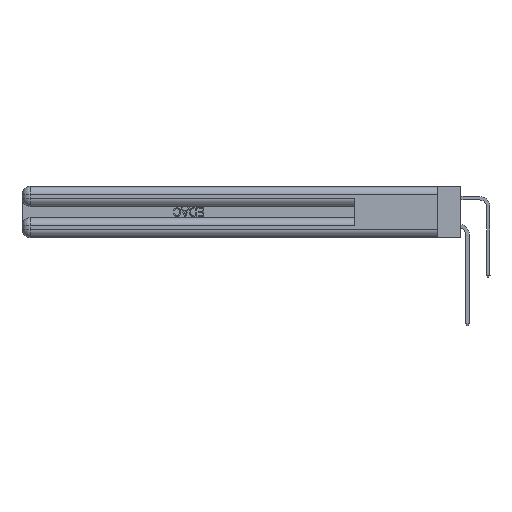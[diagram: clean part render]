
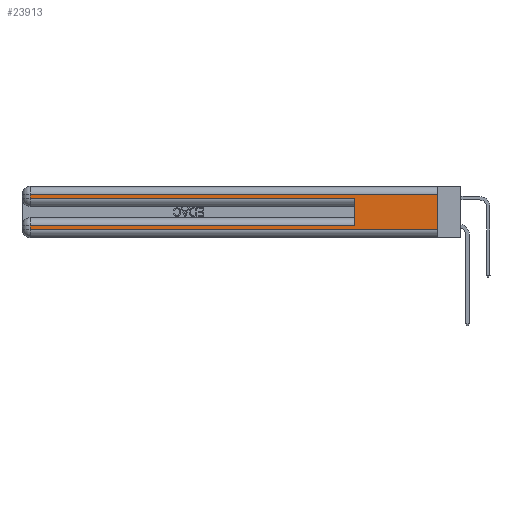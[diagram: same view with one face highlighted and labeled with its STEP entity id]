
A CAD part, left-side view. The second image highlights one B-rep face of the part: STEP entity #23913.
In plain terms, the highlighted planar face has unit normal (-1, 0, 0).
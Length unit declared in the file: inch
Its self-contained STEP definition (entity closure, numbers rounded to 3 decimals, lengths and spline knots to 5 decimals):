
#74 = LINE ( 'NONE', #33646, #19647 ) ;
#191 = CARTESIAN_POINT ( 'NONE',  ( 0., 0.6, 0.145 ) ) ;
#986 = CARTESIAN_POINT ( 'NONE',  ( 0., 2.94, 0.37 ) ) ;
#1189 = VERTEX_POINT ( 'NONE', #39160 ) ;
#1204 = LINE ( 'NONE', #39569, #29414 ) ;
#1362 = VECTOR ( 'NONE', #29673, 39.37008 ) ;
#2371 = CARTESIAN_POINT ( 'NONE',  ( 0., 0., 0.37 ) ) ;
#3102 = DIRECTION ( 'NONE',  ( 0., -1., 0. ) ) ;
#3988 = ORIENTED_EDGE ( 'NONE', *, *, #10481, .T. ) ;
#4118 = CARTESIAN_POINT ( 'NONE',  ( 0., 0., 0.37 ) ) ;
#4418 = ORIENTED_EDGE ( 'NONE', *, *, #36974, .F. ) ;
#5201 = VECTOR ( 'NONE', #18088, 39.37008 ) ;
#7004 = CARTESIAN_POINT ( 'NONE',  ( 0., 0., 0.31 ) ) ;
#8142 = VERTEX_POINT ( 'NONE', #42948 ) ;
#8772 = CARTESIAN_POINT ( 'NONE',  ( 0., 0.6, 0.285 ) ) ;
#9786 = PLANE ( 'NONE',  #21915 ) ;
#10060 = EDGE_CURVE ( 'NONE', #22740, #30011, #74, .T. ) ;
#10203 = VECTOR ( 'NONE', #3102, 39.37008 ) ;
#10481 = EDGE_CURVE ( 'NONE', #36504, #1189, #1204, .T. ) ;
#12105 = DIRECTION ( 'NONE',  ( 0., 0., -1. ) ) ;
#12320 = LINE ( 'NONE', #191, #1362 ) ;
#13488 = DIRECTION ( 'NONE',  ( 1., 0., 0. ) ) ;
#14663 = LINE ( 'NONE', #4118, #34300 ) ;
#15060 = EDGE_CURVE ( 'NONE', #8142, #37074, #45731, .T. ) ;
#15237 = DIRECTION ( 'NONE',  ( 0., 0., -1. ) ) ;
#15265 = DIRECTION ( 'NONE',  ( 0., -1., 0. ) ) ;
#16184 = EDGE_CURVE ( 'NONE', #36231, #8142, #38117, .T. ) ;
#16297 = VECTOR ( 'NONE', #12105, 39.37008 ) ;
#17117 = DIRECTION ( 'NONE',  ( 0., 0., -1. ) ) ;
#18088 = DIRECTION ( 'NONE',  ( 0., 1., 0. ) ) ;
#19647 = VECTOR ( 'NONE', #15265, 39.37008 ) ;
#21915 = AXIS2_PLACEMENT_3D ( 'NONE', #2371, #13488, #39280 ) ;
#22740 = VERTEX_POINT ( 'NONE', #27134 ) ;
#23913 = ADVANCED_FACE ( 'NONE', ( #28263 ), #9786, .F. ) ;
#27134 = CARTESIAN_POINT ( 'NONE',  ( 0., 2.94, 0.06 ) ) ;
#28263 = FACE_OUTER_BOUND ( 'NONE', #33148, .T. ) ;
#28394 = VERTEX_POINT ( 'NONE', #8772 ) ;
#28599 = LINE ( 'NONE', #28844, #10203 ) ;
#28844 = CARTESIAN_POINT ( 'NONE',  ( 0., 0., 0.285 ) ) ;
#29414 = VECTOR ( 'NONE', #35870, 39.37008 ) ;
#29673 = DIRECTION ( 'NONE',  ( 0., 0., 1. ) ) ;
#30011 = VERTEX_POINT ( 'NONE', #34278 ) ;
#30549 = ORIENTED_EDGE ( 'NONE', *, *, #16184, .T. ) ;
#32208 = ORIENTED_EDGE ( 'NONE', *, *, #15060, .T. ) ;
#33148 = EDGE_LOOP ( 'NONE', ( #46635, #30549, #32208, #41848, #4418, #3988, #36576, #47367 ) ) ;
#33646 = CARTESIAN_POINT ( 'NONE',  ( 0., 0., 0.06 ) ) ;
#33931 = CARTESIAN_POINT ( 'NONE',  ( 0., 0.6, 0.085 ) ) ;
#34278 = CARTESIAN_POINT ( 'NONE',  ( 0., 0., 0.06 ) ) ;
#34300 = VECTOR ( 'NONE', #15237, 39.37008 ) ;
#35870 = DIRECTION ( 'NONE',  ( 0., 1., 0. ) ) ;
#36231 = VERTEX_POINT ( 'NONE', #46354 ) ;
#36447 = EDGE_CURVE ( 'NONE', #36231, #30011, #14663, .T. ) ;
#36504 = VERTEX_POINT ( 'NONE', #33931 ) ;
#36576 = ORIENTED_EDGE ( 'NONE', *, *, #46703, .T. ) ;
#36974 = EDGE_CURVE ( 'NONE', #36504, #28394, #12320, .T. ) ;
#37074 = VERTEX_POINT ( 'NONE', #45018 ) ;
#38117 = LINE ( 'NONE', #7004, #5201 ) ;
#39160 = CARTESIAN_POINT ( 'NONE',  ( 0., 2.94, 0.085 ) ) ;
#39228 = CARTESIAN_POINT ( 'NONE',  ( 0., 2.94, 0.37 ) ) ;
#39280 = DIRECTION ( 'NONE',  ( 0., 0., -1. ) ) ;
#39569 = CARTESIAN_POINT ( 'NONE',  ( 0., 0., 0.085 ) ) ;
#41848 = ORIENTED_EDGE ( 'NONE', *, *, #46835, .T. ) ;
#42948 = CARTESIAN_POINT ( 'NONE',  ( 0., 2.94, 0.31 ) ) ;
#43094 = VECTOR ( 'NONE', #17117, 39.37008 ) ;
#44266 = LINE ( 'NONE', #39228, #43094 ) ;
#45018 = CARTESIAN_POINT ( 'NONE',  ( 0., 2.94, 0.285 ) ) ;
#45731 = LINE ( 'NONE', #986, #16297 ) ;
#46354 = CARTESIAN_POINT ( 'NONE',  ( 0., 0., 0.31 ) ) ;
#46635 = ORIENTED_EDGE ( 'NONE', *, *, #36447, .F. ) ;
#46703 = EDGE_CURVE ( 'NONE', #1189, #22740, #44266, .T. ) ;
#46835 = EDGE_CURVE ( 'NONE', #37074, #28394, #28599, .T. ) ;
#47367 = ORIENTED_EDGE ( 'NONE', *, *, #10060, .T. ) ;
